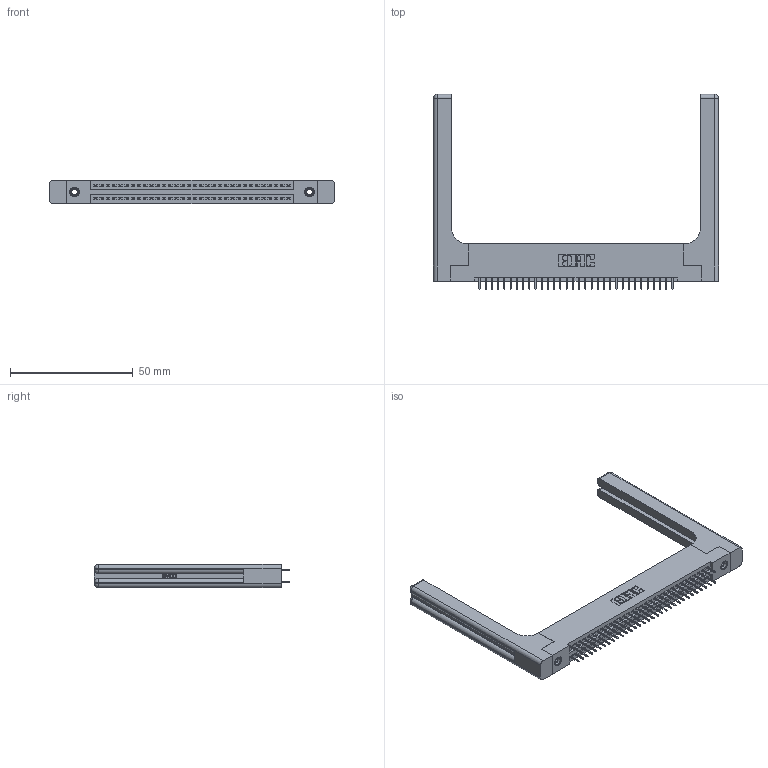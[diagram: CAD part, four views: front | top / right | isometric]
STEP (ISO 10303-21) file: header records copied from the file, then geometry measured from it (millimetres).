
FILE_DESCRIPTION (( 'STEP AP203' ), '1' );
FILE_NAME ('395-064-525-258.STEP', '2020-09-24T23:39:21', ( '' ), ( '' ), 'SwSTEP 2.0', 'SolidWorks 2020', '' );
FILE_SCHEMA (( 'CONFIG_CONTROL_DESIGN' ));
Length unit declared in the file: inch
Products named in the file (5): 345-220-058_345-220-058; 345 Part_Flush Mounting Lugs - 0.156 Dia-TH; 345-250-001_345-250-001-102; 395-064-525-258; 345-292-001_345-293-125
Assembly tree (69 placements, depth 2):
  395-064-525-258
    345 Part_Flush Mounting Lugs - 0.156 Dia-TH
    345-292-001_345-293-125  x64
    345-250-001_345-250-001-102  x2
    345-220-058_345-220-058  x2
Bounding box: 116.31 x 79.68 x 9.4 mm (x, y, z)
Volume: 19575.1 mm3; surface area: 20955.4 mm2
Topology: 69 solids, 69 shells, 3838 faces, 10799 edges, 6922 vertices
Faces by surface type: plane 2724, cylinder 1054, bspline 36, cone 12, sphere 8, torus 4
Entity records: 31710 total; most frequent: CARTESIAN_POINT 6317, ORIENTED_EDGE 5048, DIRECTION 4516, EDGE_CURVE 2524, LINE 2176, VECTOR 2176, VERTEX_POINT 1670, AXIS2_PLACEMENT_3D 1170
